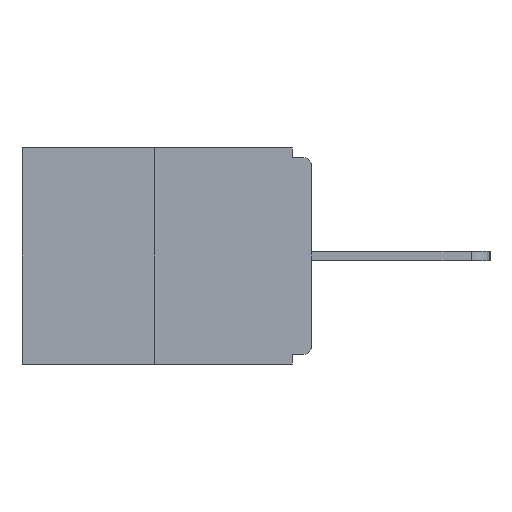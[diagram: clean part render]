
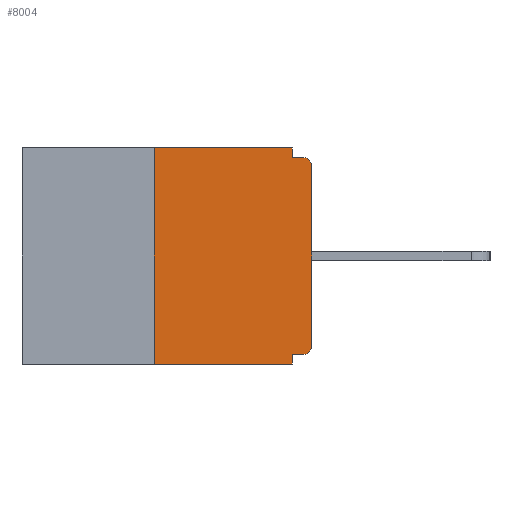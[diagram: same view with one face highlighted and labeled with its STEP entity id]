
A CAD part, left-side view. The second image highlights one B-rep face of the part: STEP entity #8004.
In plain terms, the highlighted planar face has unit normal (-1, 0, 0).
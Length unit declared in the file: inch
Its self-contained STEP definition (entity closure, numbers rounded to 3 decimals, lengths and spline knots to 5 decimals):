
#277 = LINE ( 'NONE', #11368, #2291 ) ;
#291 = ORIENTED_EDGE ( 'NONE', *, *, #7758, .T. ) ;
#684 = EDGE_CURVE ( 'NONE', #12982, #11005, #7596, .T. ) ;
#924 = CARTESIAN_POINT ( 'NONE',  ( 0., 0.46, 0. ) ) ;
#1515 = VECTOR ( 'NONE', #8733, 39.37008 ) ;
#1541 = CARTESIAN_POINT ( 'NONE',  ( 0., 0.015, -0.015 ) ) ;
#2188 = EDGE_CURVE ( 'NONE', #11005, #8663, #15595, .T. ) ;
#2202 = EDGE_CURVE ( 'NONE', #8822, #8235, #13645, .T. ) ;
#2291 = VECTOR ( 'NONE', #6549, 39.37008 ) ;
#2357 = DIRECTION ( 'NONE',  ( -1., 0., 0. ) ) ;
#2360 = CARTESIAN_POINT ( 'NONE',  ( 0., 0.031, -0.343 ) ) ;
#2427 = CARTESIAN_POINT ( 'NONE',  ( 0., 0.015, -0.03 ) ) ;
#2482 = DIRECTION ( 'NONE',  ( 0., 0., -1. ) ) ;
#2510 = CARTESIAN_POINT ( 'NONE',  ( 0., 0., 0. ) ) ;
#2646 = CARTESIAN_POINT ( 'NONE',  ( 0., 0.015, -0.313 ) ) ;
#2805 = VECTOR ( 'NONE', #4644, 39.37008 ) ;
#2984 = CARTESIAN_POINT ( 'NONE',  ( 0., 0.25, 0. ) ) ;
#3436 = EDGE_CURVE ( 'NONE', #10662, #4847, #3628, .T. ) ;
#3535 = DIRECTION ( 'NONE',  ( 0., -1., 0. ) ) ;
#3622 = CARTESIAN_POINT ( 'NONE',  ( 0., 0.031, -0.343 ) ) ;
#3628 = LINE ( 'NONE', #2360, #4631 ) ;
#3848 = DIRECTION ( 'NONE',  ( 0., -1., 0. ) ) ;
#4571 = ORIENTED_EDGE ( 'NONE', *, *, #14758, .F. ) ;
#4631 = VECTOR ( 'NONE', #14388, 39.37008 ) ;
#4644 = DIRECTION ( 'NONE',  ( 0., 0., -1. ) ) ;
#4769 = ORIENTED_EDGE ( 'NONE', *, *, #2202, .T. ) ;
#4847 = VERTEX_POINT ( 'NONE', #3622 ) ;
#5000 = EDGE_CURVE ( 'NONE', #12982, #4847, #277, .T. ) ;
#5111 = CARTESIAN_POINT ( 'NONE',  ( 0., 0.015, -0.328 ) ) ;
#5170 = ORIENTED_EDGE ( 'NONE', *, *, #3436, .F. ) ;
#5182 = EDGE_CURVE ( 'NONE', #8663, #11373, #7023, .T. ) ;
#5330 = AXIS2_PLACEMENT_3D ( 'NONE', #2427, #2357, #10831 ) ;
#5446 = VERTEX_POINT ( 'NONE', #5111 ) ;
#5597 = CIRCLE ( 'NONE', #13168, 0.015 ) ;
#5699 = ORIENTED_EDGE ( 'NONE', *, *, #12334, .F. ) ;
#5845 = PLANE ( 'NONE',  #12248 ) ;
#5949 = EDGE_LOOP ( 'NONE', ( #12974, #13995, #15200, #5170, #5699, #6147, #291, #4769, #4571, #9707 ) ) ;
#6147 = ORIENTED_EDGE ( 'NONE', *, *, #10995, .T. ) ;
#6549 = DIRECTION ( 'NONE',  ( 0., -1., 0. ) ) ;
#6964 = DIRECTION ( 'NONE',  ( 1., 0., 0. ) ) ;
#6975 = CARTESIAN_POINT ( 'NONE',  ( 0., 0.25, -0.343 ) ) ;
#7023 = LINE ( 'NONE', #11835, #2805 ) ;
#7036 = VERTEX_POINT ( 'NONE', #15563 ) ;
#7265 = LINE ( 'NONE', #13269, #11701 ) ;
#7596 = LINE ( 'NONE', #2984, #14526 ) ;
#7758 = EDGE_CURVE ( 'NONE', #7036, #8822, #8540, .T. ) ;
#8004 = ADVANCED_FACE ( 'NONE', ( #15278 ), #5845, .F. ) ;
#8054 = DIRECTION ( 'NONE',  ( 0., 0., -1. ) ) ;
#8235 = VERTEX_POINT ( 'NONE', #1541 ) ;
#8540 = LINE ( 'NONE', #2510, #11725 ) ;
#8613 = VECTOR ( 'NONE', #3535, 39.37008 ) ;
#8663 = VERTEX_POINT ( 'NONE', #12533 ) ;
#8674 = CARTESIAN_POINT ( 'NONE',  ( 0., 0.25, 0. ) ) ;
#8733 = DIRECTION ( 'NONE',  ( 0., 1., 0. ) ) ;
#8822 = VERTEX_POINT ( 'NONE', #15454 ) ;
#9707 = ORIENTED_EDGE ( 'NONE', *, *, #5182, .F. ) ;
#9840 = LINE ( 'NONE', #14671, #1515 ) ;
#10662 = VERTEX_POINT ( 'NONE', #11459 ) ;
#10831 = DIRECTION ( 'NONE',  ( 0., 0., -1. ) ) ;
#10995 = EDGE_CURVE ( 'NONE', #5446, #7036, #5597, .T. ) ;
#11005 = VERTEX_POINT ( 'NONE', #8674 ) ;
#11368 = CARTESIAN_POINT ( 'NONE',  ( 0., 0.46, -0.343 ) ) ;
#11373 = VERTEX_POINT ( 'NONE', #14516 ) ;
#11459 = CARTESIAN_POINT ( 'NONE',  ( 0., 0.031, -0.328 ) ) ;
#11701 = VECTOR ( 'NONE', #3848, 39.37008 ) ;
#11725 = VECTOR ( 'NONE', #12099, 39.37008 ) ;
#11835 = CARTESIAN_POINT ( 'NONE',  ( 0., 0.031, 0. ) ) ;
#12099 = DIRECTION ( 'NONE',  ( 0., 0., 1. ) ) ;
#12248 = AXIS2_PLACEMENT_3D ( 'NONE', #924, #6964, #8054 ) ;
#12334 = EDGE_CURVE ( 'NONE', #5446, #10662, #9840, .T. ) ;
#12415 = DIRECTION ( 'NONE',  ( 0., 0., 1. ) ) ;
#12533 = CARTESIAN_POINT ( 'NONE',  ( 0., 0.031, 0. ) ) ;
#12974 = ORIENTED_EDGE ( 'NONE', *, *, #2188, .F. ) ;
#12982 = VERTEX_POINT ( 'NONE', #6975 ) ;
#13168 = AXIS2_PLACEMENT_3D ( 'NONE', #2646, #13330, #2482 ) ;
#13269 = CARTESIAN_POINT ( 'NONE',  ( 0., 0., -0.015 ) ) ;
#13330 = DIRECTION ( 'NONE',  ( -1., 0., 0. ) ) ;
#13645 = CIRCLE ( 'NONE', #5330, 0.015 ) ;
#13995 = ORIENTED_EDGE ( 'NONE', *, *, #684, .F. ) ;
#14385 = CARTESIAN_POINT ( 'NONE',  ( 0., 0.46, 0. ) ) ;
#14388 = DIRECTION ( 'NONE',  ( 0., 0., -1. ) ) ;
#14516 = CARTESIAN_POINT ( 'NONE',  ( 0., 0.031, -0.015 ) ) ;
#14526 = VECTOR ( 'NONE', #12415, 39.37008 ) ;
#14671 = CARTESIAN_POINT ( 'NONE',  ( 0., 0., -0.328 ) ) ;
#14758 = EDGE_CURVE ( 'NONE', #11373, #8235, #7265, .T. ) ;
#15200 = ORIENTED_EDGE ( 'NONE', *, *, #5000, .T. ) ;
#15278 = FACE_OUTER_BOUND ( 'NONE', #5949, .T. ) ;
#15454 = CARTESIAN_POINT ( 'NONE',  ( 0., 0., -0.03 ) ) ;
#15563 = CARTESIAN_POINT ( 'NONE',  ( 0., 0., -0.313 ) ) ;
#15595 = LINE ( 'NONE', #14385, #8613 ) ;
